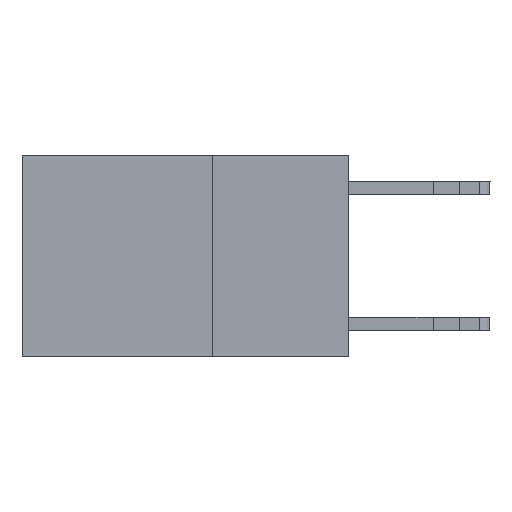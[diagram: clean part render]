
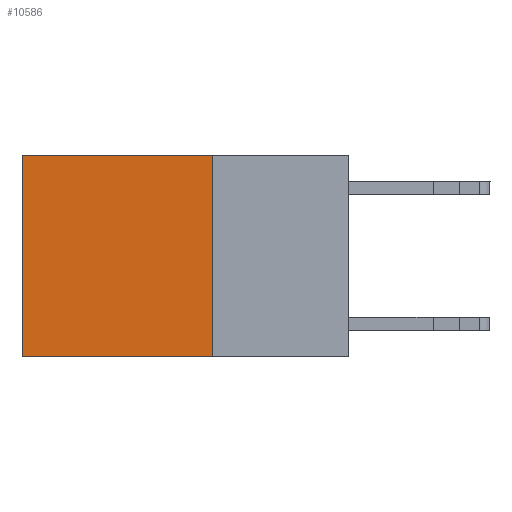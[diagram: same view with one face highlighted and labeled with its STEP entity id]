
A CAD part, left-side view. The second image highlights one B-rep face of the part: STEP entity #10586.
In plain terms, the highlighted planar face has unit normal (-1, 0, 0).
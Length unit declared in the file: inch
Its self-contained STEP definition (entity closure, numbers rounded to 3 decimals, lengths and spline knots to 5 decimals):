
#100 = ORIENTED_EDGE ( 'NONE', *, *, #10858, .T. ) ;
#1157 = EDGE_LOOP ( 'NONE', ( #100, #4940, #15692, #17963 ) ) ;
#1999 = CARTESIAN_POINT ( 'NONE',  ( 0.2625, 0.6, -0.37 ) ) ;
#2285 = DIRECTION ( 'NONE',  ( 0., 0., -1. ) ) ;
#3104 = CARTESIAN_POINT ( 'NONE',  ( 0.2625, 0.25, 0. ) ) ;
#4052 = VERTEX_POINT ( 'NONE', #1999 ) ;
#4940 = ORIENTED_EDGE ( 'NONE', *, *, #20696, .F. ) ;
#4972 = VERTEX_POINT ( 'NONE', #26654 ) ;
#5522 = CARTESIAN_POINT ( 'NONE',  ( 0.2625, 0.25, 0. ) ) ;
#7030 = DIRECTION ( 'NONE',  ( 0., 1., 0. ) ) ;
#7239 = VECTOR ( 'NONE', #2285, 39.37008 ) ;
#8719 = DIRECTION ( 'NONE',  ( 0., 1., 0. ) ) ;
#10374 = VECTOR ( 'NONE', #21120, 39.37008 ) ;
#10586 = ADVANCED_FACE ( 'NONE', ( #13745 ), #19871, .F. ) ;
#10858 = EDGE_CURVE ( 'NONE', #4972, #4052, #14033, .T. ) ;
#11354 = DIRECTION ( 'NONE',  ( 1., 0., 0. ) ) ;
#11574 = LINE ( 'NONE', #17678, #16677 ) ;
#11898 = VECTOR ( 'NONE', #8719, 39.37008 ) ;
#12188 = VERTEX_POINT ( 'NONE', #20749 ) ;
#12466 = CARTESIAN_POINT ( 'NONE',  ( 0.2625, 0.6, 0. ) ) ;
#12827 = CARTESIAN_POINT ( 'NONE',  ( 0.2625, 0.25, 0. ) ) ;
#12933 = CARTESIAN_POINT ( 'NONE',  ( 0.2625, 0.25, 0. ) ) ;
#12965 = LINE ( 'NONE', #12827, #11898 ) ;
#13745 = FACE_OUTER_BOUND ( 'NONE', #1157, .T. ) ;
#14033 = LINE ( 'NONE', #12466, #10374 ) ;
#15692 = ORIENTED_EDGE ( 'NONE', *, *, #22788, .F. ) ;
#16269 = AXIS2_PLACEMENT_3D ( 'NONE', #3104, #11354, #22404 ) ;
#16562 = VERTEX_POINT ( 'NONE', #5522 ) ;
#16677 = VECTOR ( 'NONE', #7030, 39.37008 ) ;
#17678 = CARTESIAN_POINT ( 'NONE',  ( 0.2625, 0.25, -0.37 ) ) ;
#17963 = ORIENTED_EDGE ( 'NONE', *, *, #27405, .T. ) ;
#19871 = PLANE ( 'NONE',  #16269 ) ;
#20696 = EDGE_CURVE ( 'NONE', #12188, #4052, #11574, .T. ) ;
#20749 = CARTESIAN_POINT ( 'NONE',  ( 0.2625, 0.25, -0.37 ) ) ;
#21120 = DIRECTION ( 'NONE',  ( 0., 0., -1. ) ) ;
#21450 = LINE ( 'NONE', #12933, #7239 ) ;
#22404 = DIRECTION ( 'NONE',  ( 0., 0., -1. ) ) ;
#22788 = EDGE_CURVE ( 'NONE', #16562, #12188, #21450, .T. ) ;
#26654 = CARTESIAN_POINT ( 'NONE',  ( 0.2625, 0.6, 0. ) ) ;
#27405 = EDGE_CURVE ( 'NONE', #16562, #4972, #12965, .T. ) ;
